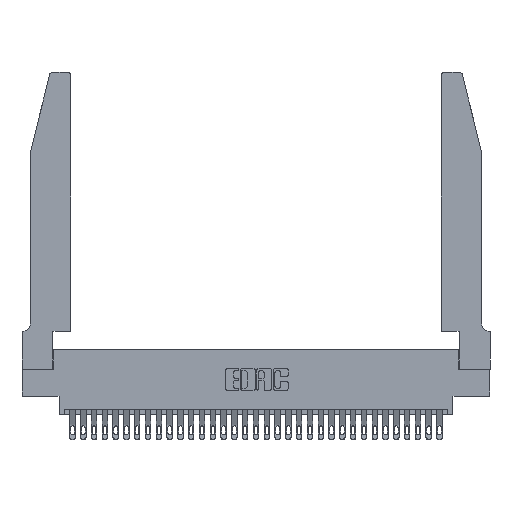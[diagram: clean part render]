
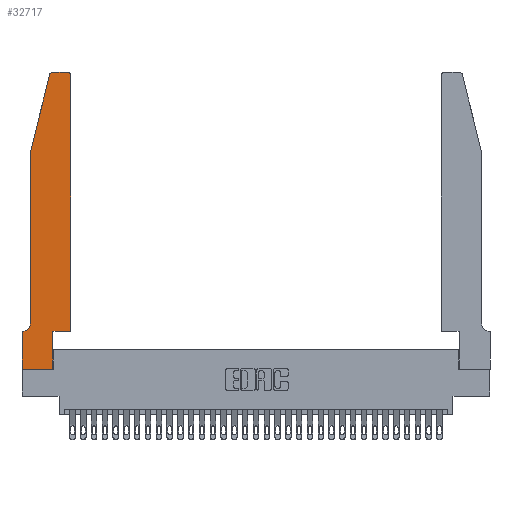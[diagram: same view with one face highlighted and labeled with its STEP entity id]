
A CAD part, top view. The second image highlights one B-rep face of the part: STEP entity #32717.
In plain terms, the highlighted planar face has unit normal (0, 0, 1).
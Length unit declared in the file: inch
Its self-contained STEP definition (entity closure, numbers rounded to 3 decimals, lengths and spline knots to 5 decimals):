
#198 = VERTEX_POINT ( 'NONE', #3313 ) ;
#1258 = CARTESIAN_POINT ( 'NONE',  ( 0.0755, 0.35, 0.37 ) ) ;
#1272 = DIRECTION ( 'NONE',  ( 0., 0., 1. ) ) ;
#1408 = CIRCLE ( 'NONE', #17900, 0.03 ) ;
#1780 = CARTESIAN_POINT ( 'NONE',  ( 0.2865, 0.35, 0.37 ) ) ;
#2195 = CARTESIAN_POINT ( 'NONE',  ( 0., 0.35, 0.37 ) ) ;
#2826 = CARTESIAN_POINT ( 'NONE',  ( 0.4505, 0.35, 0.37 ) ) ;
#3108 = CARTESIAN_POINT ( 'NONE',  ( 0.4205, 2.75, 0.37 ) ) ;
#3313 = CARTESIAN_POINT ( 'NONE',  ( 0.0055, 0.35, 0.37 ) ) ;
#3499 = CARTESIAN_POINT ( 'NONE',  ( 0.4505, 2.72, 0.37 ) ) ;
#3791 = VERTEX_POINT ( 'NONE', #20305 ) ;
#3845 = VERTEX_POINT ( 'NONE', #2195 ) ;
#3952 = DIRECTION ( 'NONE',  ( -1., 0., 0. ) ) ;
#4087 = CARTESIAN_POINT ( 'NONE',  ( 0.0755, 2., 0.37 ) ) ;
#4804 = CARTESIAN_POINT ( 'NONE',  ( 0.25487, 2.72718, 0.37 ) ) ;
#5296 = ORIENTED_EDGE ( 'NONE', *, *, #5732, .T. ) ;
#5688 = CIRCLE ( 'NONE', #18360, 0.03 ) ;
#5732 = EDGE_CURVE ( 'NONE', #32617, #15864, #15877, .T. ) ;
#6096 = DIRECTION ( 'NONE',  ( 0., 1., 0. ) ) ;
#6435 = VERTEX_POINT ( 'NONE', #21417 ) ;
#6637 = CARTESIAN_POINT ( 'NONE',  ( 0.4205, 2.72, 0.37 ) ) ;
#6874 = DIRECTION ( 'NONE',  ( 0., -1., 0. ) ) ;
#7325 = EDGE_CURVE ( 'NONE', #18147, #6435, #29036, .T. ) ;
#7511 = DIRECTION ( 'NONE',  ( 0., -1., 0. ) ) ;
#8348 = CARTESIAN_POINT ( 'NONE',  ( 0.0755, 0.42, 0.37 ) ) ;
#9256 = DIRECTION ( 'NONE',  ( 1., 0., 0. ) ) ;
#9453 = VECTOR ( 'NONE', #6874, 39.37008 ) ;
#9653 = CARTESIAN_POINT ( 'NONE',  ( 0.0055, 0.42, 0.37 ) ) ;
#9730 = VERTEX_POINT ( 'NONE', #1780 ) ;
#9902 = LINE ( 'NONE', #1258, #29713 ) ;
#10123 = CARTESIAN_POINT ( 'NONE',  ( 0.0755, 2., 0.37 ) ) ;
#10235 = EDGE_CURVE ( 'NONE', #3791, #18147, #5688, .T. ) ;
#10454 = LINE ( 'NONE', #31453, #30243 ) ;
#11356 = VECTOR ( 'NONE', #7511, 39.37008 ) ;
#12253 = DIRECTION ( 'NONE',  ( -1., 0., 0. ) ) ;
#12420 = CARTESIAN_POINT ( 'NONE',  ( 0., 0., 0.37 ) ) ;
#12458 = CARTESIAN_POINT ( 'NONE',  ( 0., 0.35, 0.37 ) ) ;
#13753 = EDGE_CURVE ( 'NONE', #18117, #15586, #14063, .T. ) ;
#14063 = LINE ( 'NONE', #15018, #26988 ) ;
#14065 = ORIENTED_EDGE ( 'NONE', *, *, #33227, .T. ) ;
#14226 = ORIENTED_EDGE ( 'NONE', *, *, #33029, .T. ) ;
#14541 = CARTESIAN_POINT ( 'NONE',  ( 0.4505, 0.35, 0.37 ) ) ;
#14612 = CARTESIAN_POINT ( 'NONE',  ( 0., 0., 0.37 ) ) ;
#15018 = CARTESIAN_POINT ( 'NONE',  ( 0., 0., 0.37 ) ) ;
#15053 = AXIS2_PLACEMENT_3D ( 'NONE', #12458, #33081, #17702 ) ;
#15190 = VERTEX_POINT ( 'NONE', #3108 ) ;
#15332 = VECTOR ( 'NONE', #19670, 39.37008 ) ;
#15586 = VERTEX_POINT ( 'NONE', #27990 ) ;
#15864 = VERTEX_POINT ( 'NONE', #3499 ) ;
#15877 = LINE ( 'NONE', #2826, #30346 ) ;
#16078 = CIRCLE ( 'NONE', #16362, 0.07 ) ;
#16362 = AXIS2_PLACEMENT_3D ( 'NONE', #9653, #27759, #12253 ) ;
#16391 = LINE ( 'NONE', #14612, #9453 ) ;
#16951 = CARTESIAN_POINT ( 'NONE',  ( 0.284, 2.72, 0.37 ) ) ;
#17018 = CARTESIAN_POINT ( 'NONE',  ( 0.4505, 0.35, 0.37 ) ) ;
#17702 = DIRECTION ( 'NONE',  ( 1., 0., 0. ) ) ;
#17891 = ORIENTED_EDGE ( 'NONE', *, *, #13753, .T. ) ;
#17900 = AXIS2_PLACEMENT_3D ( 'NONE', #6637, #24744, #9256 ) ;
#18117 = VERTEX_POINT ( 'NONE', #12420 ) ;
#18147 = VERTEX_POINT ( 'NONE', #4804 ) ;
#18360 = AXIS2_PLACEMENT_3D ( 'NONE', #16951, #1272, #19530 ) ;
#18538 = ORIENTED_EDGE ( 'NONE', *, *, #30440, .T. ) ;
#19031 = CARTESIAN_POINT ( 'NONE',  ( 0.2865, 0.35, 0.37 ) ) ;
#19507 = ORIENTED_EDGE ( 'NONE', *, *, #29358, .T. ) ;
#19530 = DIRECTION ( 'NONE',  ( 1., 0., 0. ) ) ;
#19670 = DIRECTION ( 'NONE',  ( -0.239, -0.971, 0. ) ) ;
#20305 = CARTESIAN_POINT ( 'NONE',  ( 0.284, 2.75, 0.37 ) ) ;
#20920 = EDGE_LOOP ( 'NONE', ( #18538, #26635, #21493, #27814, #26354, #25101, #14065, #17891, #14226, #19507, #5296, #32132 ) ) ;
#21417 = CARTESIAN_POINT ( 'NONE',  ( 0.0755, 2., 0.37 ) ) ;
#21493 = ORIENTED_EDGE ( 'NONE', *, *, #7325, .T. ) ;
#22047 = VECTOR ( 'NONE', #6096, 39.37008 ) ;
#22699 = LINE ( 'NONE', #17018, #29555 ) ;
#23579 = DIRECTION ( 'NONE',  ( 0., 1., 0. ) ) ;
#24073 = FACE_OUTER_BOUND ( 'NONE', #20920, .T. ) ;
#24744 = DIRECTION ( 'NONE',  ( 0., 0., 1. ) ) ;
#24906 = EDGE_CURVE ( 'NONE', #15864, #15190, #1408, .T. ) ;
#25101 = ORIENTED_EDGE ( 'NONE', *, *, #32519, .T. ) ;
#26314 = DIRECTION ( 'NONE',  ( -1., 0., 0. ) ) ;
#26354 = ORIENTED_EDGE ( 'NONE', *, *, #32088, .T. ) ;
#26635 = ORIENTED_EDGE ( 'NONE', *, *, #10235, .T. ) ;
#26988 = VECTOR ( 'NONE', #27873, 39.37008 ) ;
#27759 = DIRECTION ( 'NONE',  ( 0., 0., -1. ) ) ;
#27814 = ORIENTED_EDGE ( 'NONE', *, *, #28544, .T. ) ;
#27873 = DIRECTION ( 'NONE',  ( 1., 0., 0. ) ) ;
#27990 = CARTESIAN_POINT ( 'NONE',  ( 0.2865, 0., 0.37 ) ) ;
#28544 = EDGE_CURVE ( 'NONE', #6435, #29784, #31950, .T. ) ;
#28875 = LINE ( 'NONE', #19031, #22047 ) ;
#29036 = LINE ( 'NONE', #4087, #15332 ) ;
#29358 = EDGE_CURVE ( 'NONE', #9730, #32617, #22699, .T. ) ;
#29555 = VECTOR ( 'NONE', #32394, 39.37008 ) ;
#29713 = VECTOR ( 'NONE', #3952, 39.37008 ) ;
#29784 = VERTEX_POINT ( 'NONE', #8348 ) ;
#30243 = VECTOR ( 'NONE', #26314, 39.37008 ) ;
#30346 = VECTOR ( 'NONE', #23579, 39.37008 ) ;
#30440 = EDGE_CURVE ( 'NONE', #15190, #3791, #10454, .T. ) ;
#30505 = PLANE ( 'NONE',  #15053 ) ;
#31453 = CARTESIAN_POINT ( 'NONE',  ( 0.2605, 2.75, 0.37 ) ) ;
#31950 = LINE ( 'NONE', #10123, #11356 ) ;
#32088 = EDGE_CURVE ( 'NONE', #29784, #198, #16078, .T. ) ;
#32132 = ORIENTED_EDGE ( 'NONE', *, *, #24906, .T. ) ;
#32394 = DIRECTION ( 'NONE',  ( 1., 0., 0. ) ) ;
#32519 = EDGE_CURVE ( 'NONE', #198, #3845, #9902, .T. ) ;
#32617 = VERTEX_POINT ( 'NONE', #14541 ) ;
#32717 = ADVANCED_FACE ( 'NONE', ( #24073 ), #30505, .T. ) ;
#33029 = EDGE_CURVE ( 'NONE', #15586, #9730, #28875, .T. ) ;
#33081 = DIRECTION ( 'NONE',  ( 0., 0., 1. ) ) ;
#33227 = EDGE_CURVE ( 'NONE', #3845, #18117, #16391, .T. ) ;
